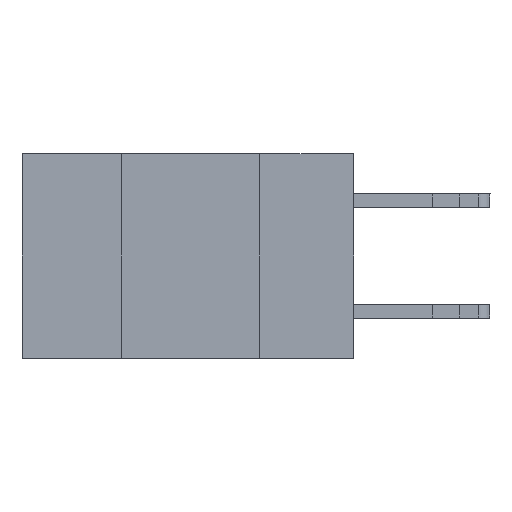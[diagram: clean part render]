
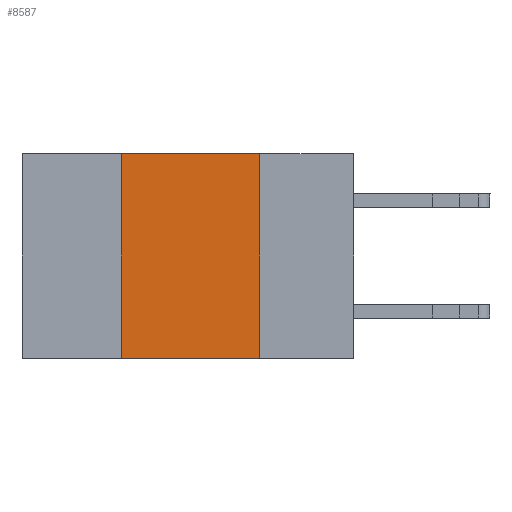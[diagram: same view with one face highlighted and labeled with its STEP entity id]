
A CAD part, left-side view. The second image highlights one B-rep face of the part: STEP entity #8587.
In plain terms, the highlighted planar face has unit normal (-1, 0, 0).
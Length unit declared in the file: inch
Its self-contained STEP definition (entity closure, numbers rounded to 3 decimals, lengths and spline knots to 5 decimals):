
#638 = LINE ( 'NONE', #8425, #21438 ) ;
#644 = EDGE_LOOP ( 'NONE', ( #15325, #34080, #33650, #27401 ) ) ;
#894 = DIRECTION ( 'NONE',  ( 0., 0., 1. ) ) ;
#1263 = EDGE_CURVE ( 'NONE', #15222, #16166, #15399, .T. ) ;
#4923 = PLANE ( 'NONE',  #9263 ) ;
#5672 = DIRECTION ( 'NONE',  ( 0., -1., 0. ) ) ;
#6843 = CARTESIAN_POINT ( 'NONE',  ( 0., 0.17, 0. ) ) ;
#7669 = DIRECTION ( 'NONE',  ( 1., 0., 0. ) ) ;
#7744 = VECTOR ( 'NONE', #894, 39.37008 ) ;
#8425 = CARTESIAN_POINT ( 'NONE',  ( 0., 0.6, 0. ) ) ;
#8587 = ADVANCED_FACE ( 'NONE', ( #23067 ), #4923, .F. ) ;
#9263 = AXIS2_PLACEMENT_3D ( 'NONE', #27787, #7669, #25214 ) ;
#9913 = CARTESIAN_POINT ( 'NONE',  ( 0., 0.42, -0.37 ) ) ;
#10796 = DIRECTION ( 'NONE',  ( 0., -1., 0. ) ) ;
#13836 = DIRECTION ( 'NONE',  ( 0., 0., -1. ) ) ;
#13984 = CARTESIAN_POINT ( 'NONE',  ( 0., 0.17, -0.37 ) ) ;
#15222 = VERTEX_POINT ( 'NONE', #9913 ) ;
#15325 = ORIENTED_EDGE ( 'NONE', *, *, #24061, .F. ) ;
#15399 = LINE ( 'NONE', #23659, #7744 ) ;
#16166 = VERTEX_POINT ( 'NONE', #36024 ) ;
#16387 = VECTOR ( 'NONE', #10796, 39.37008 ) ;
#21438 = VECTOR ( 'NONE', #5672, 39.37008 ) ;
#23067 = FACE_OUTER_BOUND ( 'NONE', #644, .T. ) ;
#23659 = CARTESIAN_POINT ( 'NONE',  ( 0., 0.42, 0. ) ) ;
#24061 = EDGE_CURVE ( 'NONE', #27357, #31188, #24196, .T. ) ;
#24196 = LINE ( 'NONE', #33512, #35612 ) ;
#25214 = DIRECTION ( 'NONE',  ( 0., 0., -1. ) ) ;
#27357 = VERTEX_POINT ( 'NONE', #6843 ) ;
#27401 = ORIENTED_EDGE ( 'NONE', *, *, #29655, .T. ) ;
#27787 = CARTESIAN_POINT ( 'NONE',  ( 0., 0.6, 0. ) ) ;
#29520 = LINE ( 'NONE', #34038, #16387 ) ;
#29655 = EDGE_CURVE ( 'NONE', #15222, #31188, #29520, .T. ) ;
#31188 = VERTEX_POINT ( 'NONE', #13984 ) ;
#33512 = CARTESIAN_POINT ( 'NONE',  ( 0., 0.17, 0. ) ) ;
#33650 = ORIENTED_EDGE ( 'NONE', *, *, #1263, .F. ) ;
#34038 = CARTESIAN_POINT ( 'NONE',  ( 0., 0.6, -0.37 ) ) ;
#34080 = ORIENTED_EDGE ( 'NONE', *, *, #35353, .F. ) ;
#35353 = EDGE_CURVE ( 'NONE', #16166, #27357, #638, .T. ) ;
#35612 = VECTOR ( 'NONE', #13836, 39.37008 ) ;
#36024 = CARTESIAN_POINT ( 'NONE',  ( 0., 0.42, 0. ) ) ;
